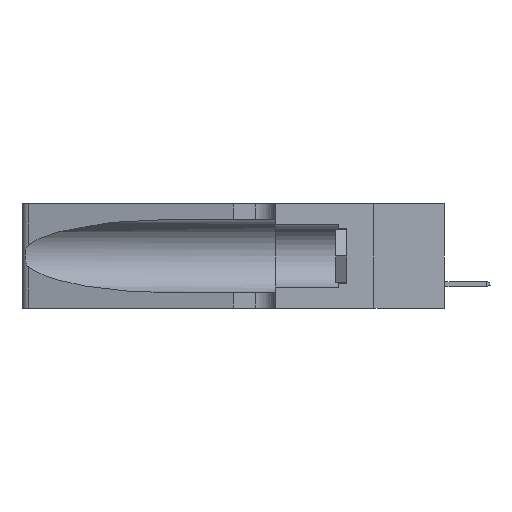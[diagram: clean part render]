
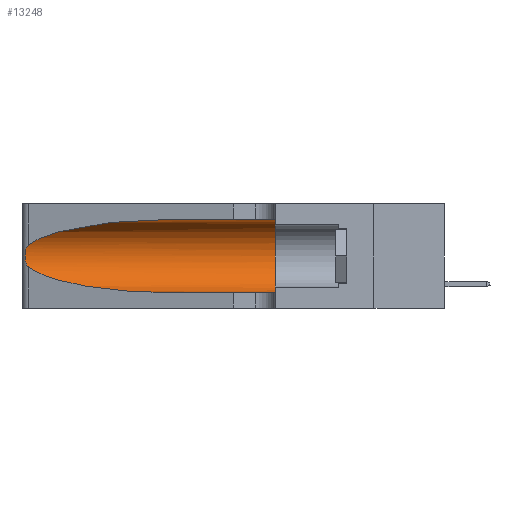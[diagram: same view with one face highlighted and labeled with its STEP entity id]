
A CAD part, left-side view. The second image highlights one B-rep face of the part: STEP entity #13248.
In plain terms, the highlighted cylindrical face has radius 3.308 mm (diameter 6.617 mm), a partial arc.
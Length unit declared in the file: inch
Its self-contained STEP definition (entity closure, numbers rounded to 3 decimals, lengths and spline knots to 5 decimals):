
#797 = CARTESIAN_POINT ( 'NONE',  ( 0.25856, 1.23593, 0.16098 ) ) ;
#2784 = CARTESIAN_POINT ( 'NONE',  ( 0.1305, 0.72297, 0.05475 ) ) ;
#3344 = VERTEX_POINT ( 'NONE', #29772 ) ;
#5046 = VERTEX_POINT ( 'NONE', #44431 ) ;
#5363 = EDGE_CURVE ( 'NONE', #30085, #10214, #26401, .T. ) ;
#6046 = DIRECTION ( 'NONE',  ( 0., -1., 0. ) ) ;
#6120 = CARTESIAN_POINT ( 'NONE',  ( 0.1305, 0.35, 0.185 ) ) ;
#7775 = CARTESIAN_POINT ( 'NONE',  ( 0.25639, 1.23184, 0.21858 ) ) ;
#9550 = CARTESIAN_POINT ( 'NONE',  ( 0.2373, 1.15595, 0.28018 ) ) ;
#10001 =( BOUNDED_CURVE ( )  B_SPLINE_CURVE ( 3, ( #43957, #26398, #29863, #30159 ),
 .UNSPECIFIED., .F., .T. ) 
 B_SPLINE_CURVE_WITH_KNOTS ( ( 4, 4 ),
 ( 3.44316, 4.71239 ),
 .UNSPECIFIED. ) 
 CURVE ( )  GEOMETRIC_REPRESENTATION_ITEM ( )  RATIONAL_B_SPLINE_CURVE ( ( 1., 0.87, 0.87, 1. ) ) 
 REPRESENTATION_ITEM ( '' )  );
#10214 = VERTEX_POINT ( 'NONE', #32533 ) ;
#10850 = CARTESIAN_POINT ( 'NONE',  ( 0.25487, 1.22718, 0.14631 ) ) ;
#11449 = CARTESIAN_POINT ( 'NONE',  ( 0.25555, 1.22994, 0.2215 ) ) ;
#12423 = EDGE_CURVE ( 'NONE', #3344, #5046, #24664, .T. ) ;
#12801 = EDGE_CURVE ( 'NONE', #3344, #29264, #14125, .T. ) ;
#13248 = ADVANCED_FACE ( 'NONE', ( #15762 ), #22813, .F. ) ;
#13676 = CIRCLE ( 'NONE', #14992, 0.13025 ) ;
#14125 = LINE ( 'NONE', #27136, #17839 ) ;
#14480 = CARTESIAN_POINT ( 'NONE',  ( 0.25789, 1.23486, 0.15765 ) ) ;
#14909 = DIRECTION ( 'NONE',  ( 0., -1., 0. ) ) ;
#14927 = CARTESIAN_POINT ( 'NONE',  ( 0.26075, 1.23896, 0.19203 ) ) ;
#14992 = AXIS2_PLACEMENT_3D ( 'NONE', #6120, #16265, #26771 ) ;
#15219 = EDGE_CURVE ( 'NONE', #29264, #10214, #13676, .T. ) ;
#15762 = FACE_OUTER_BOUND ( 'NONE', #27846, .T. ) ;
#16265 = DIRECTION ( 'NONE',  ( 0., 1., 0. ) ) ;
#17839 = VECTOR ( 'NONE', #6046, 39.37008 ) ;
#18152 = VECTOR ( 'NONE', #44489, 39.37008 ) ;
#18173 = EDGE_CURVE ( 'NONE', #30896, #30085, #10001, .T. ) ;
#18188 = CARTESIAN_POINT ( 'NONE',  ( 0.25487, 1.22718, 0.22369 ) ) ;
#18342 = CARTESIAN_POINT ( 'NONE',  ( 0.25639, 1.23186, 0.15144 ) ) ;
#20200 = CARTESIAN_POINT ( 'NONE',  ( 0.1305, 1.61858, 0.05475 ) ) ;
#20574 = ORIENTED_EDGE ( 'NONE', *, *, #15219, .F. ) ;
#21557 = CARTESIAN_POINT ( 'NONE',  ( 0.25787, 1.23484, 0.2124 ) ) ;
#22813 = CYLINDRICAL_SURFACE ( 'NONE', #24796, 0.13025 ) ;
#23178 = CARTESIAN_POINT ( 'NONE',  ( 0.1305, 0.72297, 0.31525 ) ) ;
#24664 =( BOUNDED_CURVE ( )  B_SPLINE_CURVE ( 3, ( #23178, #26682, #9550, #27120 ),
 .UNSPECIFIED., .F., .F. ) 
 B_SPLINE_CURVE_WITH_KNOTS ( ( 4, 4 ),
 ( 1.5708, 2.84003 ),
 .UNSPECIFIED. ) 
 CURVE ( )  GEOMETRIC_REPRESENTATION_ITEM ( )  RATIONAL_B_SPLINE_CURVE ( ( 1., 0.87, 0.87, 1. ) ) 
 REPRESENTATION_ITEM ( '' )  );
#24746 = ORIENTED_EDGE ( 'NONE', *, *, #12423, .T. ) ;
#24796 = AXIS2_PLACEMENT_3D ( 'NONE', #39414, #14909, #42450 ) ;
#26398 = CARTESIAN_POINT ( 'NONE',  ( 0.2373, 1.15595, 0.08982 ) ) ;
#26401 = LINE ( 'NONE', #20200, #18152 ) ;
#26682 = CARTESIAN_POINT ( 'NONE',  ( 0.18966, 0.96281, 0.31525 ) ) ;
#26771 = DIRECTION ( 'NONE',  ( 0., 0., 1. ) ) ;
#27043 = ORIENTED_EDGE ( 'NONE', *, *, #12801, .F. ) ;
#27108 = ORIENTED_EDGE ( 'NONE', *, *, #5363, .T. ) ;
#27120 = CARTESIAN_POINT ( 'NONE',  ( 0.25487, 1.22718, 0.22369 ) ) ;
#27136 = CARTESIAN_POINT ( 'NONE',  ( 0.1305, 1.61858, 0.31525 ) ) ;
#27846 = EDGE_LOOP ( 'NONE', ( #24746, #37367, #32324, #27108, #20574, #27043 ) ) ;
#28115 = CARTESIAN_POINT ( 'NONE',  ( 0.25555, 1.22993, 0.14849 ) ) ;
#29264 = VERTEX_POINT ( 'NONE', #42908 ) ;
#29772 = CARTESIAN_POINT ( 'NONE',  ( 0.1305, 0.72297, 0.31525 ) ) ;
#29863 = CARTESIAN_POINT ( 'NONE',  ( 0.18966, 0.96281, 0.05475 ) ) ;
#30085 = VERTEX_POINT ( 'NONE', #2784 ) ;
#30159 = CARTESIAN_POINT ( 'NONE',  ( 0.1305, 0.72297, 0.05475 ) ) ;
#30896 = VERTEX_POINT ( 'NONE', #39664 ) ;
#32324 = ORIENTED_EDGE ( 'NONE', *, *, #18173, .T. ) ;
#32533 = CARTESIAN_POINT ( 'NONE',  ( 0.1305, 0.35, 0.05475 ) ) ;
#35479 = CARTESIAN_POINT ( 'NONE',  ( 0.26018, 1.23835, 0.19895 ) ) ;
#35612 = CARTESIAN_POINT ( 'NONE',  ( 0.25854, 1.2359, 0.20912 ) ) ;
#37367 = ORIENTED_EDGE ( 'NONE', *, *, #43439, .T. ) ;
#39375 = B_SPLINE_CURVE_WITH_KNOTS ( 'NONE', 3,
 ( #18188, #11449, #7775, #21557, #35612, #35479, #14927, #42314, #42478, #797, #14480, #18342, #28115, #10850 ),
 .UNSPECIFIED., .F., .F.,
 ( 4, 2, 2, 2, 2, 2, 4 ),
 ( 0., 0.00027, 0.00053, 0.00107, 0.0016, 0.00187, 0.00214 ),
 .UNSPECIFIED. ) ;
#39414 = CARTESIAN_POINT ( 'NONE',  ( 0.1305, 1.61858, 0.185 ) ) ;
#39664 = CARTESIAN_POINT ( 'NONE',  ( 0.25487, 1.22718, 0.14631 ) ) ;
#42314 = CARTESIAN_POINT ( 'NONE',  ( 0.26075, 1.23896, 0.178 ) ) ;
#42450 = DIRECTION ( 'NONE',  ( 0., 0., -1. ) ) ;
#42478 = CARTESIAN_POINT ( 'NONE',  ( 0.26017, 1.23833, 0.17102 ) ) ;
#42908 = CARTESIAN_POINT ( 'NONE',  ( 0.1305, 0.35, 0.31525 ) ) ;
#43439 = EDGE_CURVE ( 'NONE', #5046, #30896, #39375, .T. ) ;
#43957 = CARTESIAN_POINT ( 'NONE',  ( 0.25487, 1.22718, 0.14631 ) ) ;
#44431 = CARTESIAN_POINT ( 'NONE',  ( 0.25487, 1.22718, 0.22369 ) ) ;
#44489 = DIRECTION ( 'NONE',  ( 0., -1., 0. ) ) ;
